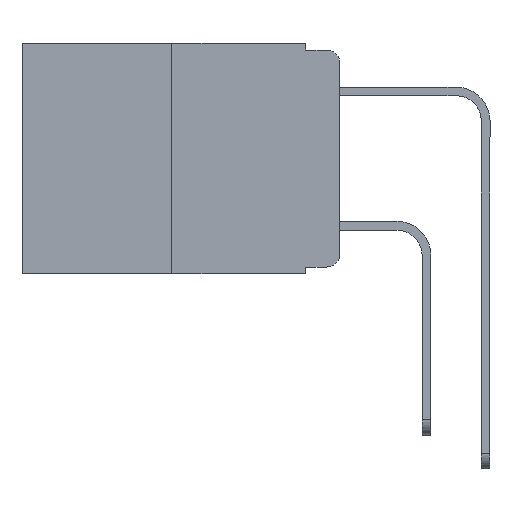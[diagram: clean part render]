
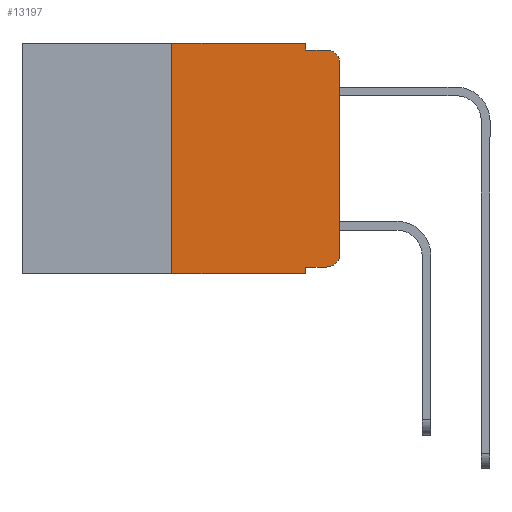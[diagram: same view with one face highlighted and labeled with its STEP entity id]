
A CAD part, left-side view. The second image highlights one B-rep face of the part: STEP entity #13197.
In plain terms, the highlighted planar face has unit normal (-1, 0, 0).
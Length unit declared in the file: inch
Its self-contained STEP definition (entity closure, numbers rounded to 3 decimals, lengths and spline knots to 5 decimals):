
#36 = CARTESIAN_POINT ( 'NONE',  ( 0., 0.25, 0. ) ) ;
#52 = CARTESIAN_POINT ( 'NONE',  ( 0., 0.473, 0. ) ) ;
#162 = VERTEX_POINT ( 'NONE', #5258 ) ;
#184 = ORIENTED_EDGE ( 'NONE', *, *, #4164, .F. ) ;
#403 = ORIENTED_EDGE ( 'NONE', *, *, #622, .T. ) ;
#440 = LINE ( 'NONE', #5331, #8855 ) ;
#578 = VERTEX_POINT ( 'NONE', #9708 ) ;
#582 = CIRCLE ( 'NONE', #11083, 0.02 ) ;
#622 = EDGE_CURVE ( 'NONE', #3978, #6105, #4630, .T. ) ;
#662 = LINE ( 'NONE', #13843, #11800 ) ;
#813 = EDGE_CURVE ( 'NONE', #7158, #162, #10143, .T. ) ;
#843 = DIRECTION ( 'NONE',  ( 0., 0., -1. ) ) ;
#1014 = CARTESIAN_POINT ( 'NONE',  ( 0., 0.051, -0.01 ) ) ;
#1148 = CARTESIAN_POINT ( 'NONE',  ( 0., 0.473, 0. ) ) ;
#1158 = EDGE_CURVE ( 'NONE', #1589, #578, #12089, .T. ) ;
#1169 = VECTOR ( 'NONE', #7111, 39.37008 ) ;
#1191 = LINE ( 'NONE', #8156, #11982 ) ;
#1354 = ORIENTED_EDGE ( 'NONE', *, *, #8541, .T. ) ;
#1502 = VECTOR ( 'NONE', #8067, 39.37008 ) ;
#1545 = FACE_OUTER_BOUND ( 'NONE', #10115, .T. ) ;
#1589 = VERTEX_POINT ( 'NONE', #1782 ) ;
#1608 = AXIS2_PLACEMENT_3D ( 'NONE', #3735, #3723, #6825 ) ;
#1782 = CARTESIAN_POINT ( 'NONE',  ( 0., 0.02, -0.333 ) ) ;
#1867 = DIRECTION ( 'NONE',  ( -1., 0., 0. ) ) ;
#1894 = EDGE_CURVE ( 'NONE', #9682, #1589, #2313, .T. ) ;
#2257 = DIRECTION ( 'NONE',  ( 0., 0., -1. ) ) ;
#2313 = LINE ( 'NONE', #4737, #4590 ) ;
#2566 = ORIENTED_EDGE ( 'NONE', *, *, #813, .F. ) ;
#3402 = EDGE_CURVE ( 'NONE', #9682, #6105, #1191, .T. ) ;
#3723 = DIRECTION ( 'NONE',  ( -1., 0., 0. ) ) ;
#3735 = CARTESIAN_POINT ( 'NONE',  ( 0., 0.02, -0.313 ) ) ;
#3846 = DIRECTION ( 'NONE',  ( 0., -1., 0. ) ) ;
#3978 = VERTEX_POINT ( 'NONE', #13021 ) ;
#4152 = LINE ( 'NONE', #8092, #1169 ) ;
#4164 = EDGE_CURVE ( 'NONE', #3978, #7158, #4152, .T. ) ;
#4590 = VECTOR ( 'NONE', #3846, 39.37008 ) ;
#4630 = LINE ( 'NONE', #13724, #9706 ) ;
#4737 = CARTESIAN_POINT ( 'NONE',  ( 0., 0.051, -0.333 ) ) ;
#5258 = CARTESIAN_POINT ( 'NONE',  ( 0., 0.051, 0. ) ) ;
#5331 = CARTESIAN_POINT ( 'NONE',  ( 0., 0.051, 0. ) ) ;
#5687 = EDGE_CURVE ( 'NONE', #162, #12259, #440, .T. ) ;
#5751 = ORIENTED_EDGE ( 'NONE', *, *, #7849, .T. ) ;
#5893 = AXIS2_PLACEMENT_3D ( 'NONE', #1148, #8832, #2257 ) ;
#6105 = VERTEX_POINT ( 'NONE', #13268 ) ;
#6433 = EDGE_CURVE ( 'NONE', #12259, #10284, #7889, .T. ) ;
#6587 = DIRECTION ( 'NONE',  ( 0., -1., 0. ) ) ;
#6652 = DIRECTION ( 'NONE',  ( 0., 0., 1. ) ) ;
#6825 = DIRECTION ( 'NONE',  ( 0., 0., -1. ) ) ;
#7111 = DIRECTION ( 'NONE',  ( 0., 0., 1. ) ) ;
#7158 = VERTEX_POINT ( 'NONE', #36 ) ;
#7544 = CARTESIAN_POINT ( 'NONE',  ( 0., 0.051, -0.333 ) ) ;
#7797 = PLANE ( 'NONE',  #5893 ) ;
#7849 = EDGE_CURVE ( 'NONE', #10456, #10284, #582, .T. ) ;
#7889 = LINE ( 'NONE', #1014, #10264 ) ;
#8067 = DIRECTION ( 'NONE',  ( 0., -1., 0. ) ) ;
#8092 = CARTESIAN_POINT ( 'NONE',  ( 0., 0.25, 0. ) ) ;
#8130 = DIRECTION ( 'NONE',  ( 0., 0., -1. ) ) ;
#8156 = CARTESIAN_POINT ( 'NONE',  ( 0., 0.051, 0. ) ) ;
#8427 = ORIENTED_EDGE ( 'NONE', *, *, #3402, .F. ) ;
#8464 = CARTESIAN_POINT ( 'NONE',  ( 0., 0.02, -0.03 ) ) ;
#8541 = EDGE_CURVE ( 'NONE', #578, #10456, #662, .T. ) ;
#8632 = CARTESIAN_POINT ( 'NONE',  ( 0., 0.02, -0.01 ) ) ;
#8719 = CARTESIAN_POINT ( 'NONE',  ( 0., 0.051, -0.01 ) ) ;
#8832 = DIRECTION ( 'NONE',  ( 1., 0., 0. ) ) ;
#8855 = VECTOR ( 'NONE', #843, 39.37008 ) ;
#9509 = DIRECTION ( 'NONE',  ( 0., 0., -1. ) ) ;
#9672 = CARTESIAN_POINT ( 'NONE',  ( 0., 0., -0.03 ) ) ;
#9682 = VERTEX_POINT ( 'NONE', #7544 ) ;
#9706 = VECTOR ( 'NONE', #10656, 39.37008 ) ;
#9708 = CARTESIAN_POINT ( 'NONE',  ( 0., 0., -0.313 ) ) ;
#9762 = ORIENTED_EDGE ( 'NONE', *, *, #1158, .T. ) ;
#10115 = EDGE_LOOP ( 'NONE', ( #1354, #5751, #12281, #12601, #2566, #184, #403, #8427, #10513, #9762 ) ) ;
#10143 = LINE ( 'NONE', #52, #1502 ) ;
#10264 = VECTOR ( 'NONE', #6587, 39.37008 ) ;
#10284 = VERTEX_POINT ( 'NONE', #8632 ) ;
#10456 = VERTEX_POINT ( 'NONE', #9672 ) ;
#10513 = ORIENTED_EDGE ( 'NONE', *, *, #1894, .T. ) ;
#10656 = DIRECTION ( 'NONE',  ( 0., -1., 0. ) ) ;
#11083 = AXIS2_PLACEMENT_3D ( 'NONE', #8464, #1867, #9509 ) ;
#11800 = VECTOR ( 'NONE', #6652, 39.37008 ) ;
#11982 = VECTOR ( 'NONE', #8130, 39.37008 ) ;
#12089 = CIRCLE ( 'NONE', #1608, 0.02 ) ;
#12259 = VERTEX_POINT ( 'NONE', #8719 ) ;
#12281 = ORIENTED_EDGE ( 'NONE', *, *, #6433, .F. ) ;
#12601 = ORIENTED_EDGE ( 'NONE', *, *, #5687, .F. ) ;
#13021 = CARTESIAN_POINT ( 'NONE',  ( 0., 0.25, -0.343 ) ) ;
#13197 = ADVANCED_FACE ( 'NONE', ( #1545 ), #7797, .F. ) ;
#13268 = CARTESIAN_POINT ( 'NONE',  ( 0., 0.051, -0.343 ) ) ;
#13724 = CARTESIAN_POINT ( 'NONE',  ( 0., 0.473, -0.343 ) ) ;
#13843 = CARTESIAN_POINT ( 'NONE',  ( 0., 0., 0. ) ) ;
